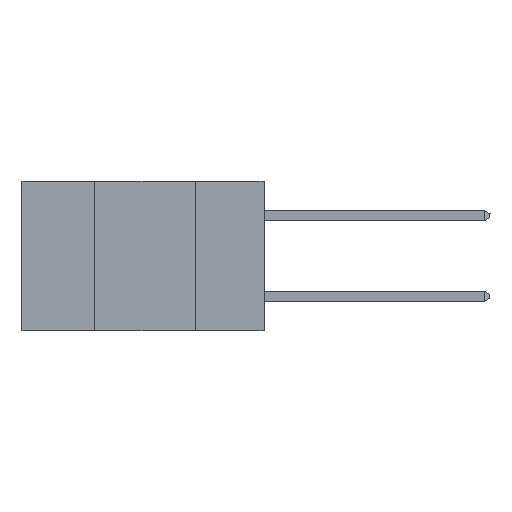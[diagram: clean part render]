
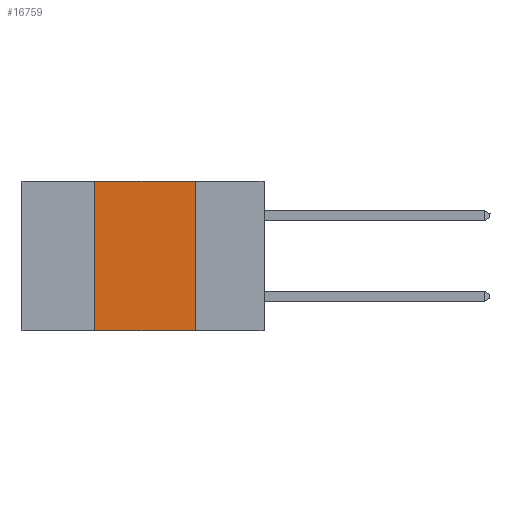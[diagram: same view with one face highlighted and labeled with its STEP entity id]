
A CAD part, left-side view. The second image highlights one B-rep face of the part: STEP entity #16759.
In plain terms, the highlighted planar face has unit normal (-1, 0, 0).
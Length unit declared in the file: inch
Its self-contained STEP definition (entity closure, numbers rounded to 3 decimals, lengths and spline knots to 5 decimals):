
#660 = CARTESIAN_POINT ( 'NONE',  ( 0., 0.6, -0.37 ) ) ;
#764 = CARTESIAN_POINT ( 'NONE',  ( 0., 0.6, 0. ) ) ;
#1940 = LINE ( 'NONE', #25255, #17783 ) ;
#2117 = VECTOR ( 'NONE', #11903, 39.37008 ) ;
#2597 = EDGE_CURVE ( 'NONE', #12092, #16597, #23972, .T. ) ;
#2857 = DIRECTION ( 'NONE',  ( 0., -1., 0. ) ) ;
#2989 = PLANE ( 'NONE',  #7425 ) ;
#3533 = CARTESIAN_POINT ( 'NONE',  ( 0., 0.42, 0. ) ) ;
#5327 = EDGE_CURVE ( 'NONE', #26191, #16597, #16551, .T. ) ;
#6738 = EDGE_CURVE ( 'NONE', #26191, #7610, #1940, .T. ) ;
#7425 = AXIS2_PLACEMENT_3D ( 'NONE', #15389, #23571, #11317 ) ;
#7610 = VERTEX_POINT ( 'NONE', #3533 ) ;
#8136 = FACE_OUTER_BOUND ( 'NONE', #10661, .T. ) ;
#10661 = EDGE_LOOP ( 'NONE', ( #26106, #14699, #11128, #22661 ) ) ;
#10955 = CARTESIAN_POINT ( 'NONE',  ( 0., 0.17, -0.37 ) ) ;
#11128 = ORIENTED_EDGE ( 'NONE', *, *, #6738, .F. ) ;
#11317 = DIRECTION ( 'NONE',  ( 0., 0., -1. ) ) ;
#11903 = DIRECTION ( 'NONE',  ( 0., 0., -1. ) ) ;
#12092 = VERTEX_POINT ( 'NONE', #13487 ) ;
#12999 = DIRECTION ( 'NONE',  ( 0., 0., 1. ) ) ;
#13487 = CARTESIAN_POINT ( 'NONE',  ( 0., 0.17, 0. ) ) ;
#14699 = ORIENTED_EDGE ( 'NONE', *, *, #25169, .F. ) ;
#15389 = CARTESIAN_POINT ( 'NONE',  ( 0., 0.6, 0. ) ) ;
#16474 = LINE ( 'NONE', #764, #26661 ) ;
#16551 = LINE ( 'NONE', #660, #21303 ) ;
#16597 = VERTEX_POINT ( 'NONE', #18999 ) ;
#16759 = ADVANCED_FACE ( 'NONE', ( #8136 ), #2989, .F. ) ;
#17249 = DIRECTION ( 'NONE',  ( 0., -1., 0. ) ) ;
#17783 = VECTOR ( 'NONE', #12999, 39.37008 ) ;
#18087 = CARTESIAN_POINT ( 'NONE',  ( 0., 0.42, -0.37 ) ) ;
#18999 = CARTESIAN_POINT ( 'NONE',  ( 0., 0.17, -0.37 ) ) ;
#21303 = VECTOR ( 'NONE', #17249, 39.37008 ) ;
#22661 = ORIENTED_EDGE ( 'NONE', *, *, #5327, .T. ) ;
#23571 = DIRECTION ( 'NONE',  ( 1., 0., 0. ) ) ;
#23972 = LINE ( 'NONE', #10955, #2117 ) ;
#25169 = EDGE_CURVE ( 'NONE', #7610, #12092, #16474, .T. ) ;
#25255 = CARTESIAN_POINT ( 'NONE',  ( 0., 0.42, -0.37 ) ) ;
#26106 = ORIENTED_EDGE ( 'NONE', *, *, #2597, .F. ) ;
#26191 = VERTEX_POINT ( 'NONE', #18087 ) ;
#26661 = VECTOR ( 'NONE', #2857, 39.37008 ) ;
